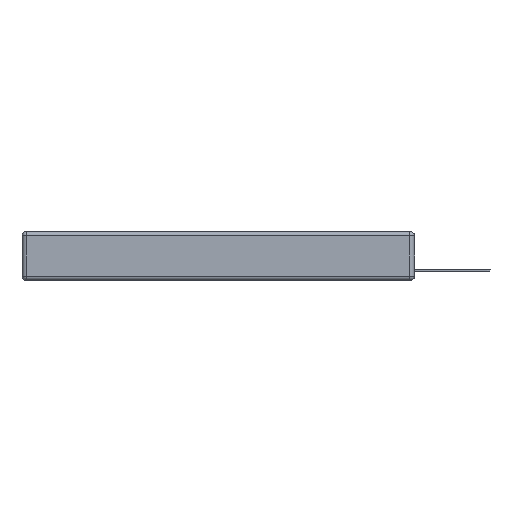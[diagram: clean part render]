
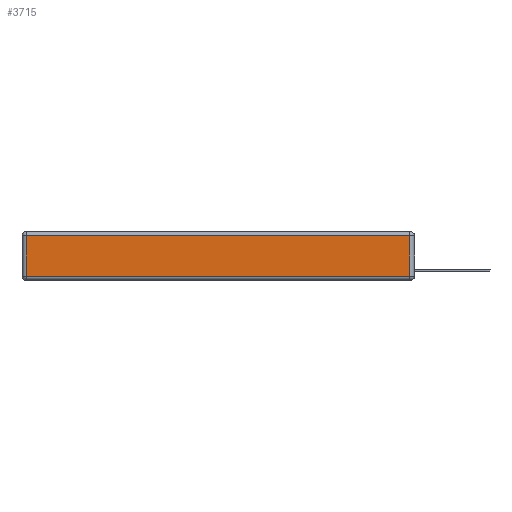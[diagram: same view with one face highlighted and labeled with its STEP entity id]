
A CAD part, left-side view. The second image highlights one B-rep face of the part: STEP entity #3715.
In plain terms, the highlighted planar face has unit normal (-1, 0, 0).
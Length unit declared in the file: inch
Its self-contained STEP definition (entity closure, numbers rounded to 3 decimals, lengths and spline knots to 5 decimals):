
#217 = VECTOR ( 'NONE', #6158, 39.37008 ) ;
#363 = LINE ( 'NONE', #2703, #217 ) ;
#395 = VECTOR ( 'NONE', #469, 39.37008 ) ;
#469 = DIRECTION ( 'NONE',  ( 0., 1., 0. ) ) ;
#815 = LINE ( 'NONE', #7096, #3038 ) ;
#1000 = LINE ( 'NONE', #4139, #395 ) ;
#2335 = VERTEX_POINT ( 'NONE', #3654 ) ;
#2703 = CARTESIAN_POINT ( 'NONE',  ( 0., 0.03, -0.343 ) ) ;
#2730 = CARTESIAN_POINT ( 'NONE',  ( 0., 0., -0.343 ) ) ;
#2889 = DIRECTION ( 'NONE',  ( -1., 0., 0. ) ) ;
#2944 = DIRECTION ( 'NONE',  ( 0., -1., 0. ) ) ;
#3038 = VECTOR ( 'NONE', #8057, 39.37008 ) ;
#3132 = EDGE_CURVE ( 'NONE', #3193, #9991, #3948, .T. ) ;
#3193 = VERTEX_POINT ( 'NONE', #11548 ) ;
#3483 = AXIS2_PLACEMENT_3D ( 'NONE', #2730, #2889, #3663 ) ;
#3654 = CARTESIAN_POINT ( 'NONE',  ( 0., 0.03, -0.03 ) ) ;
#3663 = DIRECTION ( 'NONE',  ( 0., 0., 1. ) ) ;
#3715 = ADVANCED_FACE ( 'NONE', ( #9192 ), #7635, .T. ) ;
#3948 = LINE ( 'NONE', #9510, #7684 ) ;
#4139 = CARTESIAN_POINT ( 'NONE',  ( 0., 2.75, -0.03 ) ) ;
#5458 = EDGE_CURVE ( 'NONE', #2335, #9316, #1000, .T. ) ;
#6158 = DIRECTION ( 'NONE',  ( 0., 0., 1. ) ) ;
#6218 = ORIENTED_EDGE ( 'NONE', *, *, #3132, .T. ) ;
#6686 = CARTESIAN_POINT ( 'NONE',  ( 0., 0.03, -0.313 ) ) ;
#7007 = EDGE_CURVE ( 'NONE', #9316, #3193, #815, .T. ) ;
#7096 = CARTESIAN_POINT ( 'NONE',  ( 0., 2.72, -0.343 ) ) ;
#7635 = PLANE ( 'NONE',  #3483 ) ;
#7684 = VECTOR ( 'NONE', #2944, 39.37008 ) ;
#8057 = DIRECTION ( 'NONE',  ( 0., 0., -1. ) ) ;
#8660 = CARTESIAN_POINT ( 'NONE',  ( 0., 2.72, -0.03 ) ) ;
#9192 = FACE_OUTER_BOUND ( 'NONE', #11190, .T. ) ;
#9316 = VERTEX_POINT ( 'NONE', #8660 ) ;
#9510 = CARTESIAN_POINT ( 'NONE',  ( 0., 0., -0.313 ) ) ;
#9679 = ORIENTED_EDGE ( 'NONE', *, *, #12217, .T. ) ;
#9991 = VERTEX_POINT ( 'NONE', #6686 ) ;
#10258 = ORIENTED_EDGE ( 'NONE', *, *, #5458, .T. ) ;
#11190 = EDGE_LOOP ( 'NONE', ( #6218, #9679, #10258, #11497 ) ) ;
#11497 = ORIENTED_EDGE ( 'NONE', *, *, #7007, .T. ) ;
#11548 = CARTESIAN_POINT ( 'NONE',  ( 0., 2.72, -0.313 ) ) ;
#12217 = EDGE_CURVE ( 'NONE', #9991, #2335, #363, .T. ) ;
